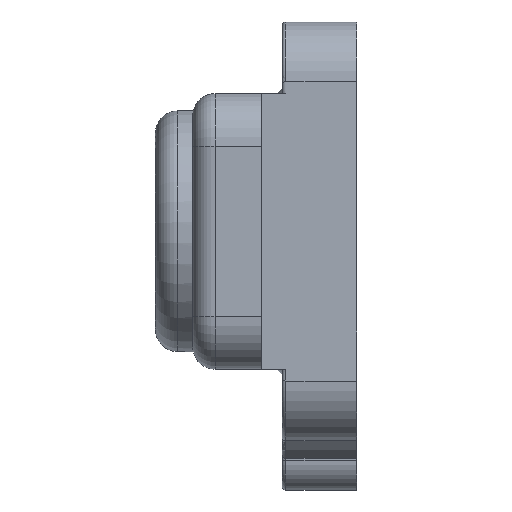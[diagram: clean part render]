
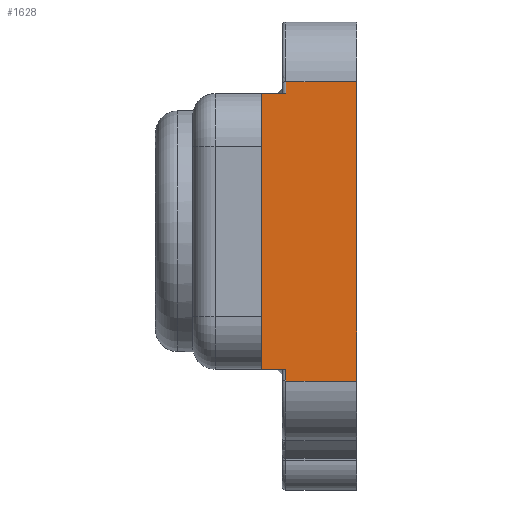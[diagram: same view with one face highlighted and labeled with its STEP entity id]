
A CAD part, front view. The second image highlights one B-rep face of the part: STEP entity #1628.
In plain terms, the highlighted planar face has unit normal (0, -1, 0).
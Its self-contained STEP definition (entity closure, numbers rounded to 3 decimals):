
#99 = EDGE_CURVE ( 'NONE', #2270, #2327, #2195, .T. ) ;
#102 = DIRECTION ( 'NONE',  ( 0., 0., -1. ) ) ;
#183 = CARTESIAN_POINT ( 'NONE',  ( -191.297, 6.367, -18.5 ) ) ;
#187 = DIRECTION ( 'NONE',  ( 1., 0., 0. ) ) ;
#212 = LINE ( 'NONE', #445, #1566 ) ;
#242 = LINE ( 'NONE', #1077, #628 ) ;
#287 = ORIENTED_EDGE ( 'NONE', *, *, #373, .T. ) ;
#373 = EDGE_CURVE ( 'NONE', #777, #907, #1772, .T. ) ;
#440 = DIRECTION ( 'NONE',  ( 0., 0., 1. ) ) ;
#445 = CARTESIAN_POINT ( 'NONE',  ( -178.497, 6.367, -20.1 ) ) ;
#481 = EDGE_CURVE ( 'NONE', #777, #2327, #1414, .T. ) ;
#522 = ORIENTED_EDGE ( 'NONE', *, *, #2119, .F. ) ;
#628 = VECTOR ( 'NONE', #2336, 1000. ) ;
#639 = DIRECTION ( 'NONE',  ( -1., 0., 0. ) ) ;
#668 = VECTOR ( 'NONE', #2427, 1000. ) ;
#692 = LINE ( 'NONE', #2290, #2607 ) ;
#777 = VERTEX_POINT ( 'NONE', #2207 ) ;
#820 = FACE_OUTER_BOUND ( 'NONE', #2112, .T. ) ;
#830 = CARTESIAN_POINT ( 'NONE',  ( -178.497, 6.367, 20.1 ) ) ;
#907 = VERTEX_POINT ( 'NONE', #183 ) ;
#962 = CARTESIAN_POINT ( 'NONE',  ( -191.297, 6.367, -1.274 ) ) ;
#1063 = ORIENTED_EDGE ( 'NONE', *, *, #2286, .F. ) ;
#1077 = CARTESIAN_POINT ( 'NONE',  ( -183.497, 6.367, -18.5 ) ) ;
#1083 = VECTOR ( 'NONE', #1849, 1000. ) ;
#1116 = CARTESIAN_POINT ( 'NONE',  ( -187.997, 6.867, 18.5 ) ) ;
#1147 = CARTESIAN_POINT ( 'NONE',  ( -178.497, 6.367, 20.1 ) ) ;
#1159 = PLANE ( 'NONE',  #1894 ) ;
#1206 = EDGE_CURVE ( 'NONE', #2401, #1270, #212, .T. ) ;
#1241 = VECTOR ( 'NONE', #1952, 1000. ) ;
#1246 = CARTESIAN_POINT ( 'NONE',  ( -178.497, 6.367, -20.1 ) ) ;
#1270 = VERTEX_POINT ( 'NONE', #2120 ) ;
#1370 = DIRECTION ( 'NONE',  ( 0., -1., 0. ) ) ;
#1414 = LINE ( 'NONE', #1613, #1445 ) ;
#1432 = EDGE_CURVE ( 'NONE', #1616, #2019, #1803, .T. ) ;
#1445 = VECTOR ( 'NONE', #187, 1000. ) ;
#1566 = VECTOR ( 'NONE', #639, 1000. ) ;
#1567 = EDGE_CURVE ( 'NONE', #2270, #2019, #1634, .T. ) ;
#1584 = DIRECTION ( 'NONE',  ( 0., 0., -1. ) ) ;
#1594 = AXIS2_PLACEMENT_3D ( 'NONE', #1116, #102, #2575 ) ;
#1613 = CARTESIAN_POINT ( 'NONE',  ( -188.497, 6.367, 18.5 ) ) ;
#1616 = VERTEX_POINT ( 'NONE', #830 ) ;
#1628 = ADVANCED_FACE ( 'NONE', ( #820 ), #1159, .T. ) ;
#1634 = LINE ( 'NONE', #2295, #1083 ) ;
#1648 = ORIENTED_EDGE ( 'NONE', *, *, #99, .T. ) ;
#1657 = ORIENTED_EDGE ( 'NONE', *, *, #481, .F. ) ;
#1772 = LINE ( 'NONE', #962, #668 ) ;
#1803 = LINE ( 'NONE', #1960, #1241 ) ;
#1849 = DIRECTION ( 'NONE',  ( 0., 0., 1. ) ) ;
#1894 = AXIS2_PLACEMENT_3D ( 'NONE', #2618, #1370, #2198 ) ;
#1906 = CARTESIAN_POINT ( 'NONE',  ( -187.997, 6.367, 20.1 ) ) ;
#1952 = DIRECTION ( 'NONE',  ( -1., 0., 0. ) ) ;
#1960 = CARTESIAN_POINT ( 'NONE',  ( -178.497, 6.367, 20.1 ) ) ;
#1982 = VERTEX_POINT ( 'NONE', #2515 ) ;
#2015 = EDGE_CURVE ( 'NONE', #1982, #907, #242, .T. ) ;
#2016 = ORIENTED_EDGE ( 'NONE', *, *, #1432, .T. ) ;
#2019 = VERTEX_POINT ( 'NONE', #1906 ) ;
#2105 = CARTESIAN_POINT ( 'NONE',  ( -187.997, 6.367, 18.5 ) ) ;
#2112 = EDGE_LOOP ( 'NONE', ( #287, #2498, #1063, #2142, #522, #2016, #2461, #1648, #1657 ) ) ;
#2119 = EDGE_CURVE ( 'NONE', #1616, #2401, #2445, .T. ) ;
#2120 = CARTESIAN_POINT ( 'NONE',  ( -187.997, 6.367, -20.1 ) ) ;
#2142 = ORIENTED_EDGE ( 'NONE', *, *, #1206, .F. ) ;
#2195 = CIRCLE ( 'NONE', #1594, 0.5 ) ;
#2198 = DIRECTION ( 'NONE',  ( 0., 0., -1. ) ) ;
#2207 = CARTESIAN_POINT ( 'NONE',  ( -191.297, 6.367, 18.5 ) ) ;
#2242 = CARTESIAN_POINT ( 'NONE',  ( -187.997, 6.367, 18.5 ) ) ;
#2270 = VERTEX_POINT ( 'NONE', #2242 ) ;
#2286 = EDGE_CURVE ( 'NONE', #1270, #1982, #692, .T. ) ;
#2290 = CARTESIAN_POINT ( 'NONE',  ( -187.997, 6.367, 20.1 ) ) ;
#2295 = CARTESIAN_POINT ( 'NONE',  ( -187.997, 6.367, 20.1 ) ) ;
#2327 = VERTEX_POINT ( 'NONE', #2105 ) ;
#2336 = DIRECTION ( 'NONE',  ( -1., 0., 0. ) ) ;
#2401 = VERTEX_POINT ( 'NONE', #1246 ) ;
#2427 = DIRECTION ( 'NONE',  ( 0., 0., -1. ) ) ;
#2445 = LINE ( 'NONE', #1147, #2648 ) ;
#2461 = ORIENTED_EDGE ( 'NONE', *, *, #1567, .F. ) ;
#2498 = ORIENTED_EDGE ( 'NONE', *, *, #2015, .F. ) ;
#2515 = CARTESIAN_POINT ( 'NONE',  ( -187.997, 6.367, -18.5 ) ) ;
#2575 = DIRECTION ( 'NONE',  ( -0.707, -0.707, 0. ) ) ;
#2607 = VECTOR ( 'NONE', #440, 1000. ) ;
#2618 = CARTESIAN_POINT ( 'NONE',  ( -188.497, 6.367, 22.767 ) ) ;
#2648 = VECTOR ( 'NONE', #1584, 1000. ) ;
